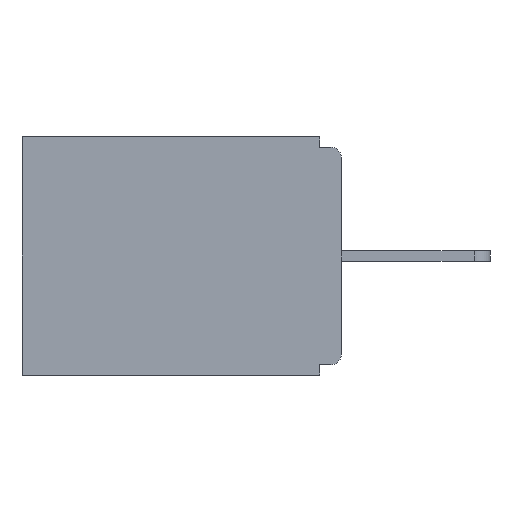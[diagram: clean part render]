
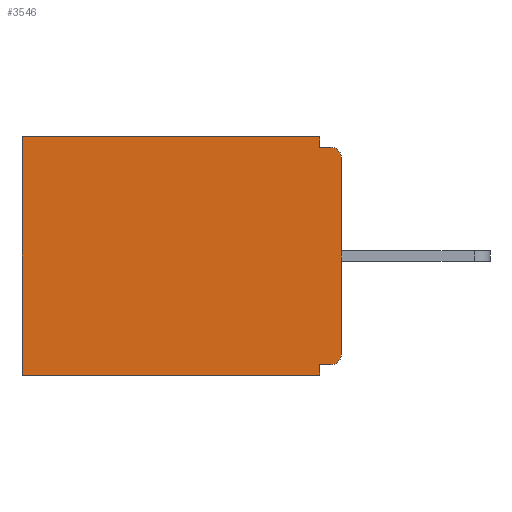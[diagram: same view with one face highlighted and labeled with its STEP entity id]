
A CAD part, left-side view. The second image highlights one B-rep face of the part: STEP entity #3546.
In plain terms, the highlighted planar face has unit normal (-1, 0, 0).
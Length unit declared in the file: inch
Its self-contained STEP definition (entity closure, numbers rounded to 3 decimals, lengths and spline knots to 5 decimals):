
#291 = CARTESIAN_POINT ( 'NONE',  ( 0.298, 0.46, -0.343 ) ) ;
#300 = CARTESIAN_POINT ( 'NONE',  ( 0.298, 0.031, -0.015 ) ) ;
#328 = AXIS2_PLACEMENT_3D ( 'NONE', #9498, #2638, #9543 ) ;
#445 = CARTESIAN_POINT ( 'NONE',  ( 0.298, 0., -0.03 ) ) ;
#462 = CARTESIAN_POINT ( 'NONE',  ( 0.298, 0.031, -0.343 ) ) ;
#486 = EDGE_CURVE ( 'NONE', #1745, #6777, #9755, .T. ) ;
#688 = CARTESIAN_POINT ( 'NONE',  ( 0.298, 0.46, 0. ) ) ;
#726 = DIRECTION ( 'NONE',  ( -1., 0., 0. ) ) ;
#773 = VECTOR ( 'NONE', #1268, 39.37008 ) ;
#1157 = EDGE_CURVE ( 'NONE', #3869, #8623, #3325, .T. ) ;
#1236 = ORIENTED_EDGE ( 'NONE', *, *, #6827, .F. ) ;
#1268 = DIRECTION ( 'NONE',  ( 0., 1., 0. ) ) ;
#1404 = CIRCLE ( 'NONE', #6395, 0.015 ) ;
#1713 = DIRECTION ( 'NONE',  ( 0., 1., 0. ) ) ;
#1745 = VERTEX_POINT ( 'NONE', #2104 ) ;
#2000 = ORIENTED_EDGE ( 'NONE', *, *, #486, .F. ) ;
#2010 = EDGE_CURVE ( 'NONE', #8623, #8888, #7609, .T. ) ;
#2104 = CARTESIAN_POINT ( 'NONE',  ( 0.298, 0.031, -0.328 ) ) ;
#2242 = CARTESIAN_POINT ( 'NONE',  ( 0.298, 0.015, -0.313 ) ) ;
#2471 = EDGE_CURVE ( 'NONE', #6178, #4947, #5205, .T. ) ;
#2638 = DIRECTION ( 'NONE',  ( 1., 0., 0. ) ) ;
#2724 = CARTESIAN_POINT ( 'NONE',  ( 0.298, 0.031, -0.343 ) ) ;
#2758 = CARTESIAN_POINT ( 'NONE',  ( 0.298, 0., -0.015 ) ) ;
#2773 = DIRECTION ( 'NONE',  ( 0., 0., -1. ) ) ;
#2801 = CARTESIAN_POINT ( 'NONE',  ( 0.298, 0.031, -0.343 ) ) ;
#2893 = EDGE_CURVE ( 'NONE', #6178, #4981, #9681, .T. ) ;
#2933 = CARTESIAN_POINT ( 'NONE',  ( 0.298, 0.015, -0.03 ) ) ;
#3212 = CARTESIAN_POINT ( 'NONE',  ( 0.298, 0.015, -0.328 ) ) ;
#3294 = ORIENTED_EDGE ( 'NONE', *, *, #2893, .F. ) ;
#3325 = LINE ( 'NONE', #5458, #4326 ) ;
#3421 = CARTESIAN_POINT ( 'NONE',  ( 0.298, 0., 0. ) ) ;
#3546 = ADVANCED_FACE ( 'NONE', ( #5560 ), #8748, .F. ) ;
#3612 = DIRECTION ( 'NONE',  ( 0., 1., 0. ) ) ;
#3738 = ORIENTED_EDGE ( 'NONE', *, *, #8975, .T. ) ;
#3869 = VERTEX_POINT ( 'NONE', #9892 ) ;
#3943 = CARTESIAN_POINT ( 'NONE',  ( 0.298, 0.46, 0. ) ) ;
#4314 = CARTESIAN_POINT ( 'NONE',  ( 0.298, 0., -0.328 ) ) ;
#4326 = VECTOR ( 'NONE', #1713, 39.37008 ) ;
#4433 = VERTEX_POINT ( 'NONE', #3212 ) ;
#4450 = DIRECTION ( 'NONE',  ( -1., 0., 0. ) ) ;
#4734 = ORIENTED_EDGE ( 'NONE', *, *, #7218, .F. ) ;
#4947 = VERTEX_POINT ( 'NONE', #8062 ) ;
#4958 = EDGE_CURVE ( 'NONE', #4433, #1745, #7457, .T. ) ;
#4981 = VERTEX_POINT ( 'NONE', #5786 ) ;
#5104 = ORIENTED_EDGE ( 'NONE', *, *, #9823, .F. ) ;
#5109 = VECTOR ( 'NONE', #9212, 39.37008 ) ;
#5169 = DIRECTION ( 'NONE',  ( 0., 0., -1. ) ) ;
#5205 = CIRCLE ( 'NONE', #7626, 0.015 ) ;
#5359 = VECTOR ( 'NONE', #2773, 39.37008 ) ;
#5458 = CARTESIAN_POINT ( 'NONE',  ( 0.298, 0., 0. ) ) ;
#5560 = FACE_OUTER_BOUND ( 'NONE', #9266, .T. ) ;
#5620 = VECTOR ( 'NONE', #7240, 39.37008 ) ;
#5786 = CARTESIAN_POINT ( 'NONE',  ( 0.298, 0., -0.313 ) ) ;
#6177 = LINE ( 'NONE', #9680, #773 ) ;
#6178 = VERTEX_POINT ( 'NONE', #445 ) ;
#6395 = AXIS2_PLACEMENT_3D ( 'NONE', #2242, #726, #6775 ) ;
#6653 = ORIENTED_EDGE ( 'NONE', *, *, #2010, .T. ) ;
#6732 = VECTOR ( 'NONE', #3612, 39.37008 ) ;
#6775 = DIRECTION ( 'NONE',  ( 0., 0., -1. ) ) ;
#6777 = VERTEX_POINT ( 'NONE', #462 ) ;
#6827 = EDGE_CURVE ( 'NONE', #3869, #7170, #8175, .T. ) ;
#7170 = VERTEX_POINT ( 'NONE', #300 ) ;
#7218 = EDGE_CURVE ( 'NONE', #7170, #4947, #8869, .T. ) ;
#7240 = DIRECTION ( 'NONE',  ( 0., 0., -1. ) ) ;
#7428 = DIRECTION ( 'NONE',  ( 0., 0., -1. ) ) ;
#7457 = LINE ( 'NONE', #4314, #6732 ) ;
#7499 = DIRECTION ( 'NONE',  ( 0., 0., -1. ) ) ;
#7609 = LINE ( 'NONE', #688, #5620 ) ;
#7626 = AXIS2_PLACEMENT_3D ( 'NONE', #2933, #4450, #5169 ) ;
#8062 = CARTESIAN_POINT ( 'NONE',  ( 0.298, 0.015, -0.015 ) ) ;
#8175 = LINE ( 'NONE', #2724, #8644 ) ;
#8623 = VERTEX_POINT ( 'NONE', #3943 ) ;
#8644 = VECTOR ( 'NONE', #7428, 39.37008 ) ;
#8748 = PLANE ( 'NONE',  #328 ) ;
#8869 = LINE ( 'NONE', #2758, #5109 ) ;
#8888 = VERTEX_POINT ( 'NONE', #291 ) ;
#8975 = EDGE_CURVE ( 'NONE', #4433, #4981, #1404, .T. ) ;
#8986 = ORIENTED_EDGE ( 'NONE', *, *, #2471, .T. ) ;
#9212 = DIRECTION ( 'NONE',  ( 0., -1., 0. ) ) ;
#9266 = EDGE_LOOP ( 'NONE', ( #8986, #4734, #1236, #9346, #6653, #5104, #2000, #9716, #3738, #3294 ) ) ;
#9346 = ORIENTED_EDGE ( 'NONE', *, *, #1157, .T. ) ;
#9456 = VECTOR ( 'NONE', #7499, 39.37008 ) ;
#9498 = CARTESIAN_POINT ( 'NONE',  ( 0.298, 0., 0. ) ) ;
#9543 = DIRECTION ( 'NONE',  ( 0., 0., -1. ) ) ;
#9680 = CARTESIAN_POINT ( 'NONE',  ( 0.298, 0., -0.343 ) ) ;
#9681 = LINE ( 'NONE', #3421, #5359 ) ;
#9716 = ORIENTED_EDGE ( 'NONE', *, *, #4958, .F. ) ;
#9755 = LINE ( 'NONE', #2801, #9456 ) ;
#9823 = EDGE_CURVE ( 'NONE', #6777, #8888, #6177, .T. ) ;
#9892 = CARTESIAN_POINT ( 'NONE',  ( 0.298, 0.031, 0. ) ) ;
